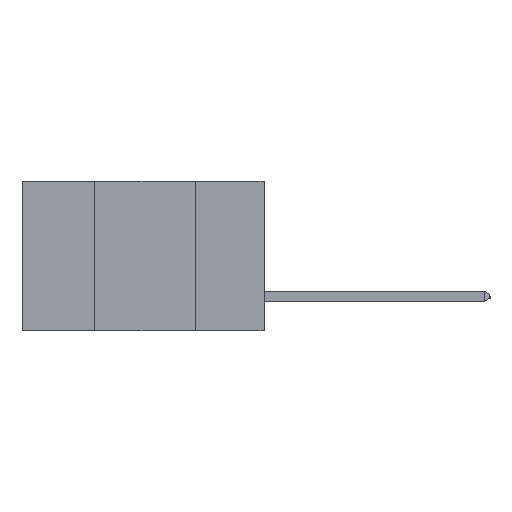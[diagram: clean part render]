
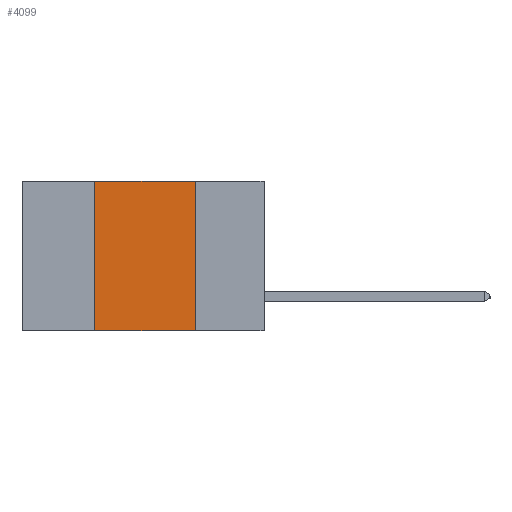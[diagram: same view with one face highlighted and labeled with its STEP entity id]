
A CAD part, left-side view. The second image highlights one B-rep face of the part: STEP entity #4099.
In plain terms, the highlighted planar face has unit normal (-1, 0, 0).
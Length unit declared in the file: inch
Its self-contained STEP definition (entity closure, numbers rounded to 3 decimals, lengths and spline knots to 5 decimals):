
#2167 = VECTOR ( 'NONE', #20751, 39.37008 ) ;
#3264 = LINE ( 'NONE', #18210, #11848 ) ;
#3383 = DIRECTION ( 'NONE',  ( 0., 0., -1. ) ) ;
#3595 = CARTESIAN_POINT ( 'NONE',  ( 0., 0.17, -0.37 ) ) ;
#3601 = ORIENTED_EDGE ( 'NONE', *, *, #10647, .F. ) ;
#4099 = ADVANCED_FACE ( 'NONE', ( #17554 ), #14380, .F. ) ;
#4667 = DIRECTION ( 'NONE',  ( 1., 0., 0. ) ) ;
#4952 = VERTEX_POINT ( 'NONE', #12765 ) ;
#5145 = VERTEX_POINT ( 'NONE', #3595 ) ;
#7478 = VECTOR ( 'NONE', #3383, 39.37008 ) ;
#7942 = CARTESIAN_POINT ( 'NONE',  ( 0., 0.6, 0. ) ) ;
#8325 = VERTEX_POINT ( 'NONE', #11141 ) ;
#8703 = DIRECTION ( 'NONE',  ( 0., 0., 1. ) ) ;
#8925 = VERTEX_POINT ( 'NONE', #18850 ) ;
#9663 = AXIS2_PLACEMENT_3D ( 'NONE', #14406, #4667, #9739 ) ;
#9739 = DIRECTION ( 'NONE',  ( 0., 0., -1. ) ) ;
#9848 = EDGE_CURVE ( 'NONE', #4952, #5145, #15936, .T. ) ;
#10647 = EDGE_CURVE ( 'NONE', #8925, #4952, #16900, .T. ) ;
#10893 = EDGE_CURVE ( 'NONE', #8325, #8925, #3264, .T. ) ;
#11141 = CARTESIAN_POINT ( 'NONE',  ( 0., 0.42, -0.37 ) ) ;
#11164 = DIRECTION ( 'NONE',  ( 0., -1., 0. ) ) ;
#11312 = CARTESIAN_POINT ( 'NONE',  ( 0., 0.6, -0.37 ) ) ;
#11848 = VECTOR ( 'NONE', #8703, 39.37008 ) ;
#11954 = EDGE_CURVE ( 'NONE', #8325, #5145, #19778, .T. ) ;
#12622 = VECTOR ( 'NONE', #11164, 39.37008 ) ;
#12678 = ORIENTED_EDGE ( 'NONE', *, *, #10893, .F. ) ;
#12765 = CARTESIAN_POINT ( 'NONE',  ( 0., 0.17, 0. ) ) ;
#14380 = PLANE ( 'NONE',  #9663 ) ;
#14406 = CARTESIAN_POINT ( 'NONE',  ( 0., 0.6, 0. ) ) ;
#14662 = CARTESIAN_POINT ( 'NONE',  ( 0., 0.17, 0. ) ) ;
#15936 = LINE ( 'NONE', #14662, #7478 ) ;
#15953 = ORIENTED_EDGE ( 'NONE', *, *, #9848, .F. ) ;
#16900 = LINE ( 'NONE', #7942, #12622 ) ;
#16947 = ORIENTED_EDGE ( 'NONE', *, *, #11954, .T. ) ;
#17554 = FACE_OUTER_BOUND ( 'NONE', #18622, .T. ) ;
#18210 = CARTESIAN_POINT ( 'NONE',  ( 0., 0.42, 0. ) ) ;
#18622 = EDGE_LOOP ( 'NONE', ( #15953, #3601, #12678, #16947 ) ) ;
#18850 = CARTESIAN_POINT ( 'NONE',  ( 0., 0.42, 0. ) ) ;
#19778 = LINE ( 'NONE', #11312, #2167 ) ;
#20751 = DIRECTION ( 'NONE',  ( 0., -1., 0. ) ) ;
